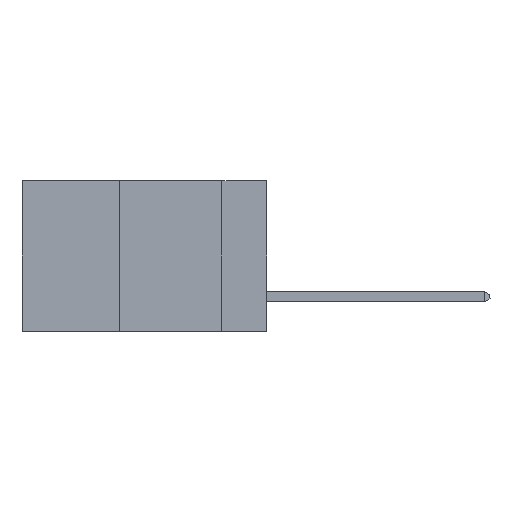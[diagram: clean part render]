
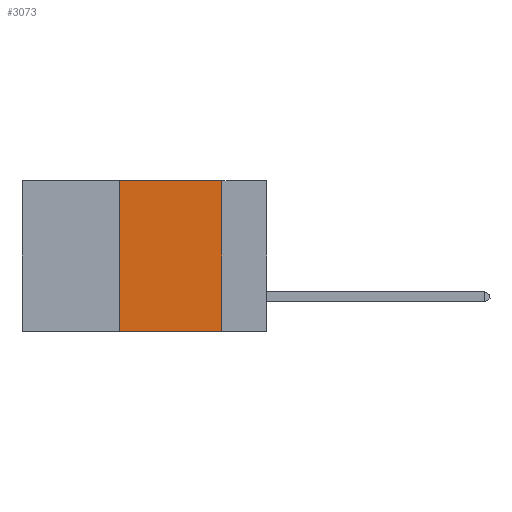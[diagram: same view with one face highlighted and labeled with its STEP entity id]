
A CAD part, left-side view. The second image highlights one B-rep face of the part: STEP entity #3073.
In plain terms, the highlighted planar face has unit normal (-1, 0, 0).
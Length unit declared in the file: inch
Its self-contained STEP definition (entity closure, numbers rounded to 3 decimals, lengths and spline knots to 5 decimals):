
#706 = ORIENTED_EDGE ( 'NONE', *, *, #12906, .F. ) ;
#2440 = VERTEX_POINT ( 'NONE', #15282 ) ;
#2452 = VERTEX_POINT ( 'NONE', #23950 ) ;
#2840 = ORIENTED_EDGE ( 'NONE', *, *, #7669, .T. ) ;
#3073 = ADVANCED_FACE ( 'NONE', ( #20040 ), #6758, .F. ) ;
#4045 = VECTOR ( 'NONE', #19464, 39.37008 ) ;
#4234 = EDGE_CURVE ( 'NONE', #13646, #2440, #13861, .T. ) ;
#4355 = CARTESIAN_POINT ( 'NONE',  ( 0., 0.11, 0. ) ) ;
#4715 = AXIS2_PLACEMENT_3D ( 'NONE', #13090, #23913, #11036 ) ;
#6758 = PLANE ( 'NONE',  #4715 ) ;
#7279 = ORIENTED_EDGE ( 'NONE', *, *, #4234, .F. ) ;
#7503 = VECTOR ( 'NONE', #11007, 39.37008 ) ;
#7669 = EDGE_CURVE ( 'NONE', #13646, #16369, #13630, .T. ) ;
#7957 = VECTOR ( 'NONE', #23798, 39.37008 ) ;
#9093 = EDGE_LOOP ( 'NONE', ( #706, #18040, #7279, #2840 ) ) ;
#10915 = CARTESIAN_POINT ( 'NONE',  ( 0., 0.6, -0.37 ) ) ;
#11007 = DIRECTION ( 'NONE',  ( 0., 0., 1. ) ) ;
#11036 = DIRECTION ( 'NONE',  ( 0., 0., -1. ) ) ;
#12051 = LINE ( 'NONE', #4355, #17121 ) ;
#12373 = EDGE_CURVE ( 'NONE', #2440, #2452, #23220, .T. ) ;
#12906 = EDGE_CURVE ( 'NONE', #2452, #16369, #12051, .T. ) ;
#13090 = CARTESIAN_POINT ( 'NONE',  ( 0., 0.6, 0. ) ) ;
#13298 = CARTESIAN_POINT ( 'NONE',  ( 0., 0.36, -0.37 ) ) ;
#13630 = LINE ( 'NONE', #10915, #7957 ) ;
#13646 = VERTEX_POINT ( 'NONE', #13298 ) ;
#13861 = LINE ( 'NONE', #19625, #7503 ) ;
#15036 = DIRECTION ( 'NONE',  ( 0., 0., -1. ) ) ;
#15143 = CARTESIAN_POINT ( 'NONE',  ( 0., 0.6, 0. ) ) ;
#15282 = CARTESIAN_POINT ( 'NONE',  ( 0., 0.36, 0. ) ) ;
#16369 = VERTEX_POINT ( 'NONE', #21038 ) ;
#17121 = VECTOR ( 'NONE', #15036, 39.37008 ) ;
#18040 = ORIENTED_EDGE ( 'NONE', *, *, #12373, .F. ) ;
#19464 = DIRECTION ( 'NONE',  ( 0., -1., 0. ) ) ;
#19625 = CARTESIAN_POINT ( 'NONE',  ( 0., 0.36, 0. ) ) ;
#20040 = FACE_OUTER_BOUND ( 'NONE', #9093, .T. ) ;
#21038 = CARTESIAN_POINT ( 'NONE',  ( 0., 0.11, -0.37 ) ) ;
#23220 = LINE ( 'NONE', #15143, #4045 ) ;
#23798 = DIRECTION ( 'NONE',  ( 0., -1., 0. ) ) ;
#23913 = DIRECTION ( 'NONE',  ( 1., 0., 0. ) ) ;
#23950 = CARTESIAN_POINT ( 'NONE',  ( 0., 0.11, 0. ) ) ;
